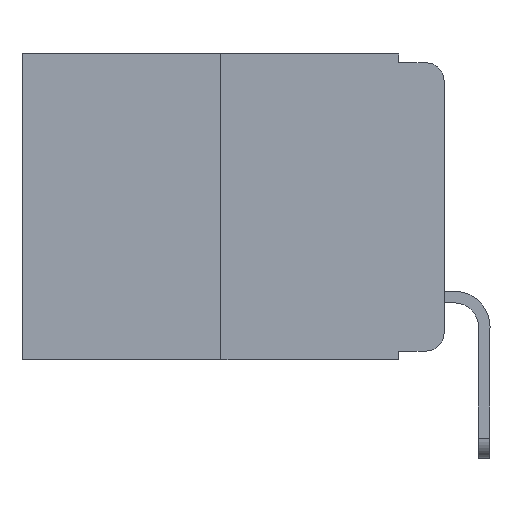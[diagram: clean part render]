
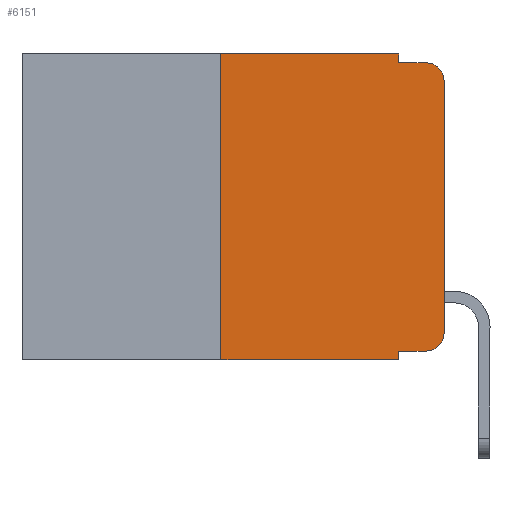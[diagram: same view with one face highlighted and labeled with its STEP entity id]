
A CAD part, left-side view. The second image highlights one B-rep face of the part: STEP entity #6151.
In plain terms, the highlighted planar face has unit normal (-1, 0, 0).
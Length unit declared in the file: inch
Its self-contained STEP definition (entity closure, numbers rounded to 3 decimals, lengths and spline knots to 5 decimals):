
#4 = ORIENTED_EDGE ( 'NONE', *, *, #5120, .F. ) ;
#186 = LINE ( 'NONE', #3053, #3284 ) ;
#655 = DIRECTION ( 'NONE',  ( 0., 0., -1. ) ) ;
#1252 = DIRECTION ( 'NONE',  ( 0., -1., 0. ) ) ;
#1365 = DIRECTION ( 'NONE',  ( 0., 0., -1. ) ) ;
#1584 = LINE ( 'NONE', #7812, #4850 ) ;
#1761 = CARTESIAN_POINT ( 'NONE',  ( 0., 0.051, -0.333 ) ) ;
#1913 = AXIS2_PLACEMENT_3D ( 'NONE', #3848, #7908, #1365 ) ;
#1918 = CIRCLE ( 'NONE', #7296, 0.02 ) ;
#1992 = EDGE_LOOP ( 'NONE', ( #7904, #8616, #4354, #6235, #4461, #4, #6252, #11148, #3755, #3361 ) ) ;
#2027 = LINE ( 'NONE', #12864, #5237 ) ;
#2399 = VERTEX_POINT ( 'NONE', #9114 ) ;
#2478 = EDGE_CURVE ( 'NONE', #8096, #9666, #4474, .T. ) ;
#2752 = VECTOR ( 'NONE', #11440, 39.37008 ) ;
#2756 = CARTESIAN_POINT ( 'NONE',  ( 0., 0.02, -0.01 ) ) ;
#2924 = EDGE_CURVE ( 'NONE', #8096, #10450, #2027, .T. ) ;
#3053 = CARTESIAN_POINT ( 'NONE',  ( 0., 0.051, -0.01 ) ) ;
#3063 = DIRECTION ( 'NONE',  ( 0., 0., -1. ) ) ;
#3215 = EDGE_CURVE ( 'NONE', #9666, #8921, #5874, .T. ) ;
#3284 = VECTOR ( 'NONE', #7324, 39.37008 ) ;
#3361 = ORIENTED_EDGE ( 'NONE', *, *, #3215, .T. ) ;
#3653 = VERTEX_POINT ( 'NONE', #8961 ) ;
#3755 = ORIENTED_EDGE ( 'NONE', *, *, #2478, .T. ) ;
#3848 = CARTESIAN_POINT ( 'NONE',  ( 0., 0.473, 0. ) ) ;
#3891 = DIRECTION ( 'NONE',  ( 0., 0., -1. ) ) ;
#4106 = FACE_OUTER_BOUND ( 'NONE', #1992, .T. ) ;
#4136 = CARTESIAN_POINT ( 'NONE',  ( 0., 0.25, 0. ) ) ;
#4156 = VERTEX_POINT ( 'NONE', #5033 ) ;
#4182 = CARTESIAN_POINT ( 'NONE',  ( 0., 0., 0. ) ) ;
#4354 = ORIENTED_EDGE ( 'NONE', *, *, #8862, .F. ) ;
#4461 = ORIENTED_EDGE ( 'NONE', *, *, #12351, .F. ) ;
#4474 = LINE ( 'NONE', #1761, #9242 ) ;
#4631 = VECTOR ( 'NONE', #9009, 39.37008 ) ;
#4703 = CARTESIAN_POINT ( 'NONE',  ( 0., 0.051, -0.333 ) ) ;
#4850 = VECTOR ( 'NONE', #1252, 39.37008 ) ;
#5031 = PLANE ( 'NONE',  #1913 ) ;
#5033 = CARTESIAN_POINT ( 'NONE',  ( 0., 0.051, 0. ) ) ;
#5120 = EDGE_CURVE ( 'NONE', #6039, #3653, #6153, .T. ) ;
#5188 = CARTESIAN_POINT ( 'NONE',  ( 0., 0.02, -0.03 ) ) ;
#5237 = VECTOR ( 'NONE', #3891, 39.37008 ) ;
#5300 = VECTOR ( 'NONE', #655, 39.37008 ) ;
#5874 = CIRCLE ( 'NONE', #10354, 0.02 ) ;
#5921 = DIRECTION ( 'NONE',  ( -1., 0., 0. ) ) ;
#5934 = CARTESIAN_POINT ( 'NONE',  ( 0., 0.02, -0.313 ) ) ;
#6039 = VERTEX_POINT ( 'NONE', #9599 ) ;
#6151 = ADVANCED_FACE ( 'NONE', ( #4106 ), #5031, .F. ) ;
#6153 = LINE ( 'NONE', #4136, #2752 ) ;
#6224 = DIRECTION ( 'NONE',  ( 0., 0., -1. ) ) ;
#6235 = ORIENTED_EDGE ( 'NONE', *, *, #9003, .F. ) ;
#6252 = ORIENTED_EDGE ( 'NONE', *, *, #7159, .T. ) ;
#6277 = VERTEX_POINT ( 'NONE', #2756 ) ;
#6415 = VECTOR ( 'NONE', #11291, 39.37008 ) ;
#6422 = EDGE_CURVE ( 'NONE', #8921, #8639, #7270, .T. ) ;
#7159 = EDGE_CURVE ( 'NONE', #6039, #10450, #8812, .T. ) ;
#7270 = LINE ( 'NONE', #4182, #4631 ) ;
#7296 = AXIS2_PLACEMENT_3D ( 'NONE', #5188, #11373, #6224 ) ;
#7324 = DIRECTION ( 'NONE',  ( 0., -1., 0. ) ) ;
#7812 = CARTESIAN_POINT ( 'NONE',  ( 0., 0.473, 0. ) ) ;
#7892 = CARTESIAN_POINT ( 'NONE',  ( 0., 0.473, -0.343 ) ) ;
#7904 = ORIENTED_EDGE ( 'NONE', *, *, #6422, .T. ) ;
#7908 = DIRECTION ( 'NONE',  ( 1., 0., 0. ) ) ;
#8096 = VERTEX_POINT ( 'NONE', #4703 ) ;
#8588 = EDGE_CURVE ( 'NONE', #8639, #6277, #1918, .T. ) ;
#8606 = CARTESIAN_POINT ( 'NONE',  ( 0., 0.051, -0.343 ) ) ;
#8616 = ORIENTED_EDGE ( 'NONE', *, *, #8588, .T. ) ;
#8639 = VERTEX_POINT ( 'NONE', #9765 ) ;
#8812 = LINE ( 'NONE', #7892, #6415 ) ;
#8862 = EDGE_CURVE ( 'NONE', #2399, #6277, #186, .T. ) ;
#8921 = VERTEX_POINT ( 'NONE', #11605 ) ;
#8961 = CARTESIAN_POINT ( 'NONE',  ( 0., 0.25, 0. ) ) ;
#9003 = EDGE_CURVE ( 'NONE', #4156, #2399, #12010, .T. ) ;
#9007 = CARTESIAN_POINT ( 'NONE',  ( 0., 0.02, -0.333 ) ) ;
#9009 = DIRECTION ( 'NONE',  ( 0., 0., 1. ) ) ;
#9114 = CARTESIAN_POINT ( 'NONE',  ( 0., 0.051, -0.01 ) ) ;
#9242 = VECTOR ( 'NONE', #10582, 39.37008 ) ;
#9599 = CARTESIAN_POINT ( 'NONE',  ( 0., 0.25, -0.343 ) ) ;
#9666 = VERTEX_POINT ( 'NONE', #9007 ) ;
#9765 = CARTESIAN_POINT ( 'NONE',  ( 0., 0., -0.03 ) ) ;
#10354 = AXIS2_PLACEMENT_3D ( 'NONE', #5934, #5921, #3063 ) ;
#10450 = VERTEX_POINT ( 'NONE', #8606 ) ;
#10582 = DIRECTION ( 'NONE',  ( 0., -1., 0. ) ) ;
#11148 = ORIENTED_EDGE ( 'NONE', *, *, #2924, .F. ) ;
#11291 = DIRECTION ( 'NONE',  ( 0., -1., 0. ) ) ;
#11373 = DIRECTION ( 'NONE',  ( -1., 0., 0. ) ) ;
#11440 = DIRECTION ( 'NONE',  ( 0., 0., 1. ) ) ;
#11605 = CARTESIAN_POINT ( 'NONE',  ( 0., 0., -0.313 ) ) ;
#12010 = LINE ( 'NONE', #12462, #5300 ) ;
#12351 = EDGE_CURVE ( 'NONE', #3653, #4156, #1584, .T. ) ;
#12462 = CARTESIAN_POINT ( 'NONE',  ( 0., 0.051, 0. ) ) ;
#12864 = CARTESIAN_POINT ( 'NONE',  ( 0., 0.051, 0. ) ) ;
